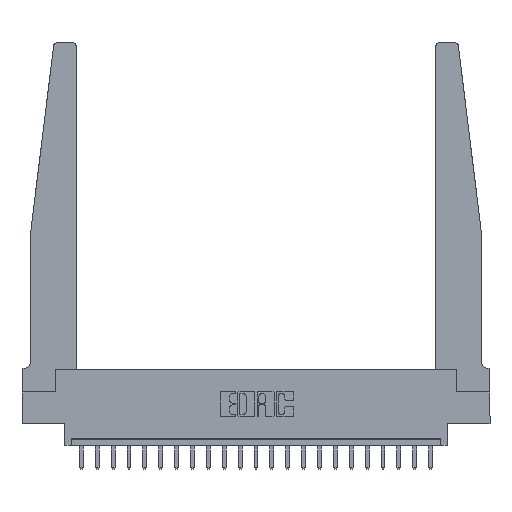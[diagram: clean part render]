
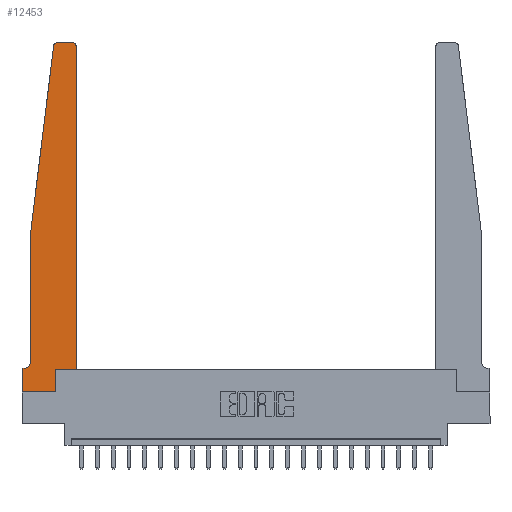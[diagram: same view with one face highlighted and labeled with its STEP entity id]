
A CAD part, top view. The second image highlights one B-rep face of the part: STEP entity #12453.
In plain terms, the highlighted planar face has unit normal (0, 0, 1).
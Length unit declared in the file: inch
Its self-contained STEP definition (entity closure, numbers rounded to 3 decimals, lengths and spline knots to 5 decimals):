
#75 = VECTOR ( 'NONE', #3922, 39.37008 ) ;
#95 = CARTESIAN_POINT ( 'NONE',  ( 0.015, 0.1875, 0.37 ) ) ;
#1179 = CIRCLE ( 'NONE', #4227, 0.05 ) ;
#1630 = DIRECTION ( 'NONE',  ( -0.122, -0.992, 0. ) ) ;
#1738 = VERTEX_POINT ( 'NONE', #10483 ) ;
#1826 = DIRECTION ( 'NONE',  ( 0., 0., 1. ) ) ;
#1838 = ORIENTED_EDGE ( 'NONE', *, *, #9510, .T. ) ;
#1888 = DIRECTION ( 'NONE',  ( 0., 0., 1. ) ) ;
#2097 = CARTESIAN_POINT ( 'NONE',  ( 0.425, 2.72, 0.37 ) ) ;
#2297 = VERTEX_POINT ( 'NONE', #3240 ) ;
#2700 = DIRECTION ( 'NONE',  ( 0., 1., 0. ) ) ;
#3240 = CARTESIAN_POINT ( 'NONE',  ( 0.065, 0.2375, 0.37 ) ) ;
#3377 = EDGE_CURVE ( 'NONE', #10312, #8418, #13588, .T. ) ;
#3461 = FACE_OUTER_BOUND ( 'NONE', #16568, .T. ) ;
#3583 = ORIENTED_EDGE ( 'NONE', *, *, #7154, .T. ) ;
#3687 = DIRECTION ( 'NONE',  ( 1., 0., 0. ) ) ;
#3762 = DIRECTION ( 'NONE',  ( -1., 0., 0. ) ) ;
#3764 = EDGE_CURVE ( 'NONE', #7710, #10312, #20142, .T. ) ;
#3877 = ORIENTED_EDGE ( 'NONE', *, *, #4311, .T. ) ;
#3922 = DIRECTION ( 'NONE',  ( 0., -1., 0. ) ) ;
#4012 = AXIS2_PLACEMENT_3D ( 'NONE', #9460, #14433, #19485 ) ;
#4227 = AXIS2_PLACEMENT_3D ( 'NONE', #18891, #5527, #12349 ) ;
#4311 = EDGE_CURVE ( 'NONE', #18770, #20373, #6110, .T. ) ;
#5076 = CARTESIAN_POINT ( 'NONE',  ( 0., 0., 0.37 ) ) ;
#5103 = DIRECTION ( 'NONE',  ( 1., 0., 0. ) ) ;
#5261 = CARTESIAN_POINT ( 'NONE',  ( 0.27653, 2.72, 0.37 ) ) ;
#5336 = DIRECTION ( 'NONE',  ( 1., 0., 0. ) ) ;
#5527 = DIRECTION ( 'NONE',  ( 0., 0., -1. ) ) ;
#5599 = CARTESIAN_POINT ( 'NONE',  ( 0.065, 1.25, 0.37 ) ) ;
#5822 = ORIENTED_EDGE ( 'NONE', *, *, #18705, .T. ) ;
#6089 = CARTESIAN_POINT ( 'NONE',  ( 0.425, 0.18, 0.37 ) ) ;
#6110 = LINE ( 'NONE', #5076, #8501 ) ;
#6422 = DIRECTION ( 'NONE',  ( -1., 0., 0. ) ) ;
#6768 = CARTESIAN_POINT ( 'NONE',  ( 0., 0.1875, 0.37 ) ) ;
#7118 = ORIENTED_EDGE ( 'NONE', *, *, #3377, .T. ) ;
#7154 = EDGE_CURVE ( 'NONE', #10176, #7710, #14190, .T. ) ;
#7710 = VERTEX_POINT ( 'NONE', #2097 ) ;
#8068 = VECTOR ( 'NONE', #6422, 39.37008 ) ;
#8418 = VERTEX_POINT ( 'NONE', #20749 ) ;
#8501 = VECTOR ( 'NONE', #3687, 39.37008 ) ;
#8844 = EDGE_CURVE ( 'NONE', #15504, #14329, #16586, .T. ) ;
#8941 = CARTESIAN_POINT ( 'NONE',  ( 0., 0., 0.37 ) ) ;
#9208 = VERTEX_POINT ( 'NONE', #16161 ) ;
#9249 = CARTESIAN_POINT ( 'NONE',  ( 0.2605, 0.18, 0.37 ) ) ;
#9460 = CARTESIAN_POINT ( 'NONE',  ( 0., 0.1875, 0.37 ) ) ;
#9510 = EDGE_CURVE ( 'NONE', #9208, #10176, #10457, .T. ) ;
#9832 = ORIENTED_EDGE ( 'NONE', *, *, #12503, .T. ) ;
#10107 = LINE ( 'NONE', #5599, #75 ) ;
#10168 = CARTESIAN_POINT ( 'NONE',  ( 0., 0., 0.37 ) ) ;
#10176 = VERTEX_POINT ( 'NONE', #6089 ) ;
#10312 = VERTEX_POINT ( 'NONE', #19886 ) ;
#10457 = LINE ( 'NONE', #15262, #19383 ) ;
#10479 = CARTESIAN_POINT ( 'NONE',  ( 0.065, 1.25, 0.37 ) ) ;
#10483 = CARTESIAN_POINT ( 'NONE',  ( 0.24675, 2.72367, 0.37 ) ) ;
#10643 = ORIENTED_EDGE ( 'NONE', *, *, #16369, .T. ) ;
#10907 = DIRECTION ( 'NONE',  ( 0., 1., 0. ) ) ;
#11177 = EDGE_CURVE ( 'NONE', #19884, #2297, #10107, .T. ) ;
#11841 = CARTESIAN_POINT ( 'NONE',  ( 0.065, 1.25, 0.37 ) ) ;
#11869 = ORIENTED_EDGE ( 'NONE', *, *, #15489, .T. ) ;
#11929 = CARTESIAN_POINT ( 'NONE',  ( 0.2605, 0., 0.37 ) ) ;
#12145 = ORIENTED_EDGE ( 'NONE', *, *, #11177, .T. ) ;
#12349 = DIRECTION ( 'NONE',  ( -1., 0., 0. ) ) ;
#12453 = ADVANCED_FACE ( 'NONE', ( #3461 ), #16214, .T. ) ;
#12503 = EDGE_CURVE ( 'NONE', #20373, #9208, #14531, .T. ) ;
#12592 = VECTOR ( 'NONE', #10907, 39.37008 ) ;
#13579 = DIRECTION ( 'NONE',  ( 0., -1., 0. ) ) ;
#13588 = LINE ( 'NONE', #18812, #20694 ) ;
#13847 = CARTESIAN_POINT ( 'NONE',  ( 0.395, 2.72, 0.37 ) ) ;
#14143 = ORIENTED_EDGE ( 'NONE', *, *, #16372, .T. ) ;
#14190 = LINE ( 'NONE', #19037, #12592 ) ;
#14329 = VERTEX_POINT ( 'NONE', #6768 ) ;
#14433 = DIRECTION ( 'NONE',  ( 0., 0., 1. ) ) ;
#14531 = LINE ( 'NONE', #9249, #14790 ) ;
#14790 = VECTOR ( 'NONE', #2700, 39.37008 ) ;
#15262 = CARTESIAN_POINT ( 'NONE',  ( 0.425, 0.18, 0.37 ) ) ;
#15489 = EDGE_CURVE ( 'NONE', #1738, #19884, #16831, .T. ) ;
#15504 = VERTEX_POINT ( 'NONE', #95 ) ;
#16161 = CARTESIAN_POINT ( 'NONE',  ( 0.2605, 0.18, 0.37 ) ) ;
#16214 = PLANE ( 'NONE',  #4012 ) ;
#16369 = EDGE_CURVE ( 'NONE', #14329, #18770, #20846, .T. ) ;
#16372 = EDGE_CURVE ( 'NONE', #8418, #1738, #16378, .T. ) ;
#16378 = CIRCLE ( 'NONE', #18895, 0.03 ) ;
#16568 = EDGE_LOOP ( 'NONE', ( #7118, #14143, #11869, #12145, #5822, #17250, #10643, #3877, #9832, #1838, #3583, #21549 ) ) ;
#16586 = LINE ( 'NONE', #21779, #8068 ) ;
#16831 = LINE ( 'NONE', #11841, #16907 ) ;
#16907 = VECTOR ( 'NONE', #1630, 39.37008 ) ;
#17250 = ORIENTED_EDGE ( 'NONE', *, *, #8844, .T. ) ;
#18705 = EDGE_CURVE ( 'NONE', #2297, #15504, #1179, .T. ) ;
#18770 = VERTEX_POINT ( 'NONE', #8941 ) ;
#18812 = CARTESIAN_POINT ( 'NONE',  ( 0.25, 2.75, 0.37 ) ) ;
#18891 = CARTESIAN_POINT ( 'NONE',  ( 0.015, 0.2375, 0.37 ) ) ;
#18895 = AXIS2_PLACEMENT_3D ( 'NONE', #5261, #1826, #20414 ) ;
#19037 = CARTESIAN_POINT ( 'NONE',  ( 0.425, 0.18, 0.37 ) ) ;
#19383 = VECTOR ( 'NONE', #5103, 39.37008 ) ;
#19485 = DIRECTION ( 'NONE',  ( 1., 0., 0. ) ) ;
#19884 = VERTEX_POINT ( 'NONE', #10479 ) ;
#19886 = CARTESIAN_POINT ( 'NONE',  ( 0.395, 2.75, 0.37 ) ) ;
#20005 = AXIS2_PLACEMENT_3D ( 'NONE', #13847, #1888, #5336 ) ;
#20142 = CIRCLE ( 'NONE', #20005, 0.03 ) ;
#20373 = VERTEX_POINT ( 'NONE', #11929 ) ;
#20414 = DIRECTION ( 'NONE',  ( 1., 0., 0. ) ) ;
#20694 = VECTOR ( 'NONE', #3762, 39.37008 ) ;
#20749 = CARTESIAN_POINT ( 'NONE',  ( 0.27653, 2.75, 0.37 ) ) ;
#20846 = LINE ( 'NONE', #10168, #21358 ) ;
#21358 = VECTOR ( 'NONE', #13579, 39.37008 ) ;
#21549 = ORIENTED_EDGE ( 'NONE', *, *, #3764, .T. ) ;
#21779 = CARTESIAN_POINT ( 'NONE',  ( 0.065, 0.1875, 0.37 ) ) ;
